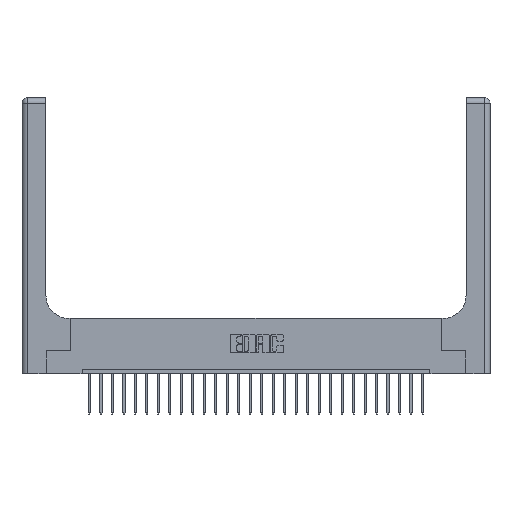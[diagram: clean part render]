
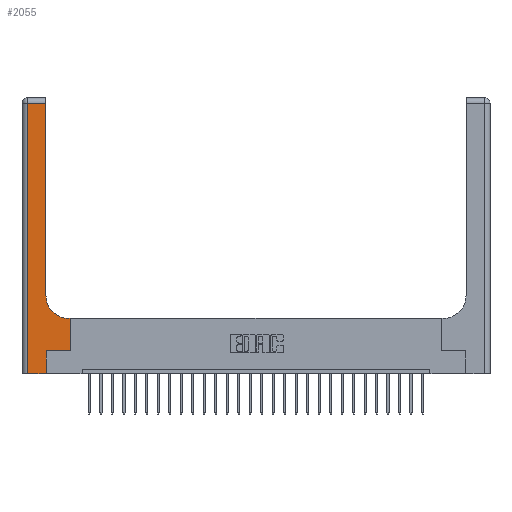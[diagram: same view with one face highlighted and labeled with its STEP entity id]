
A CAD part, top view. The second image highlights one B-rep face of the part: STEP entity #2055.
In plain terms, the highlighted planar face has unit normal (0, 0, 1).
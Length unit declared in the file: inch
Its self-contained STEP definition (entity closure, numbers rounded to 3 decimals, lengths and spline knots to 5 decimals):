
#50 = VECTOR ( 'NONE', #12639, 39.37008 ) ;
#428 = VERTEX_POINT ( 'NONE', #20696 ) ;
#582 = VECTOR ( 'NONE', #1802, 39.37008 ) ;
#787 = LINE ( 'NONE', #20675, #14835 ) ;
#877 = CARTESIAN_POINT ( 'NONE',  ( 0.51, 0.6, 0.37 ) ) ;
#1103 = DIRECTION ( 'NONE',  ( -1., 0., 0. ) ) ;
#1107 = VERTEX_POINT ( 'NONE', #8199 ) ;
#1281 = LINE ( 'NONE', #12567, #14101 ) ;
#1802 = DIRECTION ( 'NONE',  ( 0., -1., 0. ) ) ;
#1928 = CARTESIAN_POINT ( 'NONE',  ( 0.51, 0.85, 0.37 ) ) ;
#2055 = ADVANCED_FACE ( 'NONE', ( #5161 ), #7101, .F. ) ;
#2878 = ORIENTED_EDGE ( 'NONE', *, *, #16851, .T. ) ;
#3002 = ORIENTED_EDGE ( 'NONE', *, *, #17428, .T. ) ;
#3027 = CARTESIAN_POINT ( 'NONE',  ( 0.528, 0.25, 0.37 ) ) ;
#3197 = VERTEX_POINT ( 'NONE', #877 ) ;
#3285 = CARTESIAN_POINT ( 'NONE',  ( 0.265, 0., 0.37 ) ) ;
#3878 = ORIENTED_EDGE ( 'NONE', *, *, #23866, .T. ) ;
#4526 = VERTEX_POINT ( 'NONE', #17996 ) ;
#4663 = CARTESIAN_POINT ( 'NONE',  ( 0., 0., 0.37 ) ) ;
#5025 = DIRECTION ( 'NONE',  ( 0., 0., -1. ) ) ;
#5161 = FACE_OUTER_BOUND ( 'NONE', #21207, .T. ) ;
#5195 = DIRECTION ( 'NONE',  ( 0., 1., 0. ) ) ;
#5676 = VECTOR ( 'NONE', #25704, 39.37008 ) ;
#5744 = VERTEX_POINT ( 'NONE', #3027 ) ;
#6323 = AXIS2_PLACEMENT_3D ( 'NONE', #1928, #17507, #9625 ) ;
#6649 = VERTEX_POINT ( 'NONE', #15768 ) ;
#6667 = VECTOR ( 'NONE', #22078, 39.37008 ) ;
#7101 = PLANE ( 'NONE',  #24548 ) ;
#7112 = CARTESIAN_POINT ( 'NONE',  ( 0.06, 0., 0.37 ) ) ;
#7636 = ORIENTED_EDGE ( 'NONE', *, *, #15853, .T. ) ;
#8077 = VECTOR ( 'NONE', #23732, 39.37008 ) ;
#8199 = CARTESIAN_POINT ( 'NONE',  ( 0.265, 0.25, 0.37 ) ) ;
#8302 = ORIENTED_EDGE ( 'NONE', *, *, #22938, .T. ) ;
#8563 = ORIENTED_EDGE ( 'NONE', *, *, #13140, .T. ) ;
#9625 = DIRECTION ( 'NONE',  ( 1., 0., 0. ) ) ;
#10120 = ORIENTED_EDGE ( 'NONE', *, *, #21621, .T. ) ;
#11161 = CARTESIAN_POINT ( 'NONE',  ( 0., 3., 0.37 ) ) ;
#11200 = LINE ( 'NONE', #15277, #20255 ) ;
#11685 = LINE ( 'NONE', #13145, #5676 ) ;
#11855 = LINE ( 'NONE', #15920, #6667 ) ;
#12567 = CARTESIAN_POINT ( 'NONE',  ( 0.528, 0.25, 0.37 ) ) ;
#12639 = DIRECTION ( 'NONE',  ( 1., 0., 0. ) ) ;
#13119 = CARTESIAN_POINT ( 'NONE',  ( 0.26, 0.85, 0.37 ) ) ;
#13140 = EDGE_CURVE ( 'NONE', #5744, #428, #1281, .T. ) ;
#13145 = CARTESIAN_POINT ( 'NONE',  ( 0.26, 3., 0.37 ) ) ;
#14101 = VECTOR ( 'NONE', #17250, 39.37008 ) ;
#14835 = VECTOR ( 'NONE', #22777, 39.37008 ) ;
#15123 = EDGE_CURVE ( 'NONE', #428, #3197, #22023, .T. ) ;
#15277 = CARTESIAN_POINT ( 'NONE',  ( 0.265, 0., 0.37 ) ) ;
#15768 = CARTESIAN_POINT ( 'NONE',  ( 0.26, 2.94, 0.37 ) ) ;
#15784 = ORIENTED_EDGE ( 'NONE', *, *, #18718, .T. ) ;
#15815 = LINE ( 'NONE', #21827, #582 ) ;
#15853 = EDGE_CURVE ( 'NONE', #4526, #25464, #15815, .T. ) ;
#15920 = CARTESIAN_POINT ( 'NONE',  ( 0., 2.94, 0.37 ) ) ;
#16851 = EDGE_CURVE ( 'NONE', #1107, #5744, #787, .T. ) ;
#17250 = DIRECTION ( 'NONE',  ( 0., 1., 0. ) ) ;
#17428 = EDGE_CURVE ( 'NONE', #22166, #1107, #11200, .T. ) ;
#17507 = DIRECTION ( 'NONE',  ( 0., 0., -1. ) ) ;
#17612 = CIRCLE ( 'NONE', #6323, 0.25 ) ;
#17996 = CARTESIAN_POINT ( 'NONE',  ( 0.06, 2.94, 0.37 ) ) ;
#18529 = ORIENTED_EDGE ( 'NONE', *, *, #15123, .T. ) ;
#18718 = EDGE_CURVE ( 'NONE', #20275, #6649, #11685, .T. ) ;
#20037 = CARTESIAN_POINT ( 'NONE',  ( 0.26, 0.6, 0.37 ) ) ;
#20255 = VECTOR ( 'NONE', #5195, 39.37008 ) ;
#20275 = VERTEX_POINT ( 'NONE', #13119 ) ;
#20675 = CARTESIAN_POINT ( 'NONE',  ( 0.265, 0.25, 0.37 ) ) ;
#20696 = CARTESIAN_POINT ( 'NONE',  ( 0.528, 0.6, 0.37 ) ) ;
#21207 = EDGE_LOOP ( 'NONE', ( #15784, #10120, #7636, #8302, #3002, #2878, #8563, #18529, #3878 ) ) ;
#21621 = EDGE_CURVE ( 'NONE', #6649, #4526, #11855, .T. ) ;
#21827 = CARTESIAN_POINT ( 'NONE',  ( 0.06, 3., 0.37 ) ) ;
#22023 = LINE ( 'NONE', #20037, #8077 ) ;
#22078 = DIRECTION ( 'NONE',  ( -1., 0., 0. ) ) ;
#22166 = VERTEX_POINT ( 'NONE', #3285 ) ;
#22598 = LINE ( 'NONE', #4663, #50 ) ;
#22777 = DIRECTION ( 'NONE',  ( 1., 0., 0. ) ) ;
#22938 = EDGE_CURVE ( 'NONE', #25464, #22166, #22598, .T. ) ;
#23732 = DIRECTION ( 'NONE',  ( -1., 0., 0. ) ) ;
#23866 = EDGE_CURVE ( 'NONE', #3197, #20275, #17612, .T. ) ;
#24548 = AXIS2_PLACEMENT_3D ( 'NONE', #11161, #5025, #1103 ) ;
#25464 = VERTEX_POINT ( 'NONE', #7112 ) ;
#25704 = DIRECTION ( 'NONE',  ( 0., 1., 0. ) ) ;
